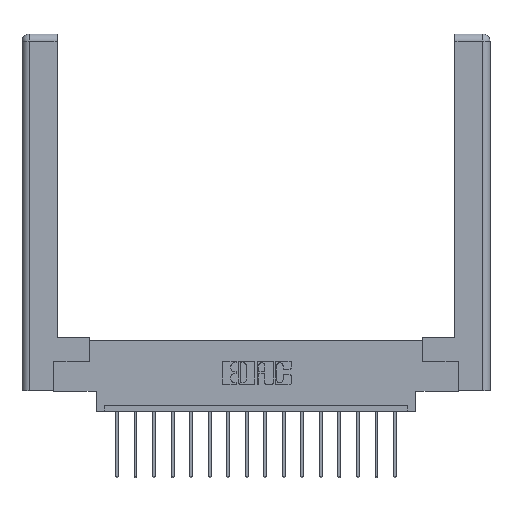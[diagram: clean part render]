
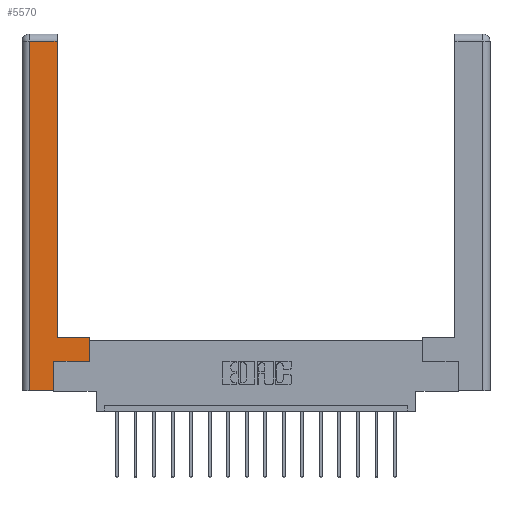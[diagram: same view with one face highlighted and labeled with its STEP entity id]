
A CAD part, top view. The second image highlights one B-rep face of the part: STEP entity #5570.
In plain terms, the highlighted planar face has unit normal (0, 0, 1).
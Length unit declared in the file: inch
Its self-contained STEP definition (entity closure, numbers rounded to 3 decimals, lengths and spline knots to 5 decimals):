
#48 = PLANE ( 'NONE',  #16308 ) ;
#106 = DIRECTION ( 'NONE',  ( 0., 0., -1. ) ) ;
#276 = CARTESIAN_POINT ( 'NONE',  ( 0.0615, 0., 0. ) ) ;
#361 = VERTEX_POINT ( 'NONE', #12745 ) ;
#462 = ORIENTED_EDGE ( 'NONE', *, *, #7285, .T. ) ;
#646 = EDGE_CURVE ( 'NONE', #11978, #3685, #9184, .T. ) ;
#757 = LINE ( 'NONE', #14381, #6426 ) ;
#1209 = CARTESIAN_POINT ( 'NONE',  ( 0.265, 0., 0. ) ) ;
#1249 = ORIENTED_EDGE ( 'NONE', *, *, #15050, .T. ) ;
#1554 = ORIENTED_EDGE ( 'NONE', *, *, #6193, .T. ) ;
#1595 = CARTESIAN_POINT ( 'NONE',  ( 0.295, 2.94, 0. ) ) ;
#1787 = ORIENTED_EDGE ( 'NONE', *, *, #2967, .T. ) ;
#2172 = VECTOR ( 'NONE', #10618, 39.37008 ) ;
#2254 = ORIENTED_EDGE ( 'NONE', *, *, #14506, .T. ) ;
#2605 = LINE ( 'NONE', #15065, #7617 ) ;
#2967 = EDGE_CURVE ( 'NONE', #361, #11978, #7394, .T. ) ;
#3271 = CARTESIAN_POINT ( 'NONE',  ( 0.265, 0.245, 0. ) ) ;
#3312 = ORIENTED_EDGE ( 'NONE', *, *, #14125, .T. ) ;
#3424 = CARTESIAN_POINT ( 'NONE',  ( 0.295, 0.45, 0. ) ) ;
#3601 = CARTESIAN_POINT ( 'NONE',  ( 0.565, 0.45, 0. ) ) ;
#3685 = VERTEX_POINT ( 'NONE', #8410 ) ;
#4207 = CARTESIAN_POINT ( 'NONE',  ( 0.265, 0.245, 0. ) ) ;
#4860 = VERTEX_POINT ( 'NONE', #7465 ) ;
#5375 = DIRECTION ( 'NONE',  ( 1., 0., 0. ) ) ;
#5570 = ADVANCED_FACE ( 'NONE', ( #8850 ), #48, .F. ) ;
#5703 = CARTESIAN_POINT ( 'NONE',  ( 0., 0., 0. ) ) ;
#6184 = VERTEX_POINT ( 'NONE', #3271 ) ;
#6193 = EDGE_CURVE ( 'NONE', #6184, #361, #757, .T. ) ;
#6214 = DIRECTION ( 'NONE',  ( -1., 0., 0. ) ) ;
#6426 = VECTOR ( 'NONE', #15897, 39.37008 ) ;
#6915 = VECTOR ( 'NONE', #5375, 39.37008 ) ;
#6994 = DIRECTION ( 'NONE',  ( -1., 0., 0. ) ) ;
#7285 = EDGE_CURVE ( 'NONE', #14232, #6184, #15199, .T. ) ;
#7394 = LINE ( 'NONE', #3601, #2172 ) ;
#7465 = CARTESIAN_POINT ( 'NONE',  ( 0.0615, 2.94, 0. ) ) ;
#7466 = DIRECTION ( 'NONE',  ( 0., -1., 0. ) ) ;
#7583 = VECTOR ( 'NONE', #7466, 39.37008 ) ;
#7614 = CARTESIAN_POINT ( 'NONE',  ( 0.0615, 0., 0. ) ) ;
#7617 = VECTOR ( 'NONE', #12102, 39.37008 ) ;
#8300 = CARTESIAN_POINT ( 'NONE',  ( 0.265, 0., 0. ) ) ;
#8410 = CARTESIAN_POINT ( 'NONE',  ( 0.295, 0.45, 0. ) ) ;
#8457 = DIRECTION ( 'NONE',  ( 0., 1., 0. ) ) ;
#8469 = LINE ( 'NONE', #276, #7583 ) ;
#8485 = LINE ( 'NONE', #17673, #16136 ) ;
#8850 = FACE_OUTER_BOUND ( 'NONE', #15680, .T. ) ;
#9184 = LINE ( 'NONE', #3424, #15107 ) ;
#9489 = VERTEX_POINT ( 'NONE', #7614 ) ;
#10552 = VERTEX_POINT ( 'NONE', #1595 ) ;
#10618 = DIRECTION ( 'NONE',  ( 0., 1., 0. ) ) ;
#11729 = LINE ( 'NONE', #1209, #6915 ) ;
#11910 = ORIENTED_EDGE ( 'NONE', *, *, #15158, .T. ) ;
#11978 = VERTEX_POINT ( 'NONE', #12281 ) ;
#12102 = DIRECTION ( 'NONE',  ( 0., 1., 0. ) ) ;
#12281 = CARTESIAN_POINT ( 'NONE',  ( 0.565, 0.45, 0. ) ) ;
#12745 = CARTESIAN_POINT ( 'NONE',  ( 0.565, 0.245, 0. ) ) ;
#14125 = EDGE_CURVE ( 'NONE', #3685, #10552, #2605, .T. ) ;
#14232 = VERTEX_POINT ( 'NONE', #8300 ) ;
#14381 = CARTESIAN_POINT ( 'NONE',  ( 0.565, 0.245, 0. ) ) ;
#14506 = EDGE_CURVE ( 'NONE', #10552, #4860, #8485, .T. ) ;
#14742 = DIRECTION ( 'NONE',  ( -1., 0., 0. ) ) ;
#15050 = EDGE_CURVE ( 'NONE', #4860, #9489, #8469, .T. ) ;
#15065 = CARTESIAN_POINT ( 'NONE',  ( 0.295, 3., 0. ) ) ;
#15107 = VECTOR ( 'NONE', #6214, 39.37008 ) ;
#15158 = EDGE_CURVE ( 'NONE', #9489, #14232, #11729, .T. ) ;
#15199 = LINE ( 'NONE', #4207, #15434 ) ;
#15434 = VECTOR ( 'NONE', #8457, 39.37008 ) ;
#15680 = EDGE_LOOP ( 'NONE', ( #3312, #2254, #1249, #11910, #462, #1554, #1787, #15872 ) ) ;
#15872 = ORIENTED_EDGE ( 'NONE', *, *, #646, .T. ) ;
#15897 = DIRECTION ( 'NONE',  ( 1., 0., 0. ) ) ;
#16136 = VECTOR ( 'NONE', #14742, 39.37008 ) ;
#16308 = AXIS2_PLACEMENT_3D ( 'NONE', #5703, #106, #6994 ) ;
#17673 = CARTESIAN_POINT ( 'NONE',  ( 0.0615, 2.94, 0. ) ) ;
